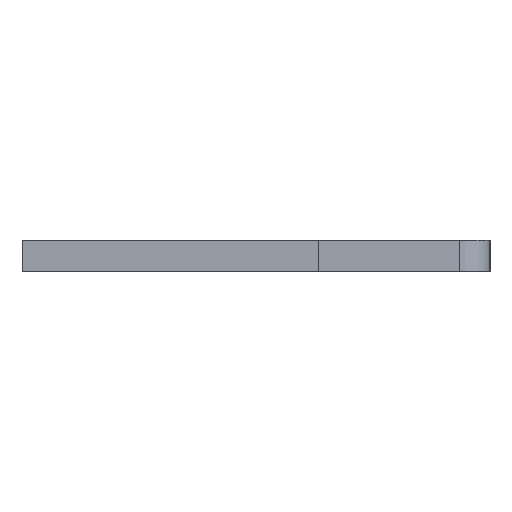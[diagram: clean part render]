
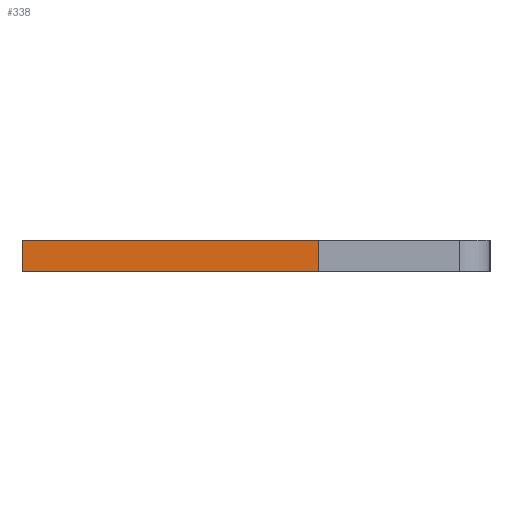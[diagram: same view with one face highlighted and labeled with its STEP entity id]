
A CAD part, left-side view. The second image highlights one B-rep face of the part: STEP entity #338.
In plain terms, the highlighted face is planar.
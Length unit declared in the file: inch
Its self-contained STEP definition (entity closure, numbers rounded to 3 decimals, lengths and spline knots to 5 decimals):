
#32 = LINE ( 'NONE', #143, #63 ) ;
#63 = VECTOR ( 'NONE', #862, 39.37008 ) ;
#90 = PLANE ( 'NONE',  #142 ) ;
#142 = AXIS2_PLACEMENT_3D ( 'NONE', #460, #455, #638 ) ;
#143 = CARTESIAN_POINT ( 'NONE',  ( 0.01, -0.04, -0.04 ) ) ;
#186 = CARTESIAN_POINT ( 'NONE',  ( 0.01, 0.15, -0.04 ) ) ;
#319 = VERTEX_POINT ( 'NONE', #376 ) ;
#338 = ADVANCED_FACE ( 'NONE', ( #926 ), #90, .F. ) ;
#369 = VERTEX_POINT ( 'NONE', #722 ) ;
#376 = CARTESIAN_POINT ( 'NONE',  ( -0.01, -0.04, -0.04 ) ) ;
#380 = CARTESIAN_POINT ( 'NONE',  ( 0.01, 0.15, -0.04 ) ) ;
#418 = CARTESIAN_POINT ( 'NONE',  ( -0.01, 0.15, -0.04 ) ) ;
#434 = LINE ( 'NONE', #1019, #910 ) ;
#449 = VERTEX_POINT ( 'NONE', #186 ) ;
#455 = DIRECTION ( 'NONE',  ( 0., 0., 1. ) ) ;
#460 = CARTESIAN_POINT ( 'NONE',  ( 0.01, 0.15, -0.04 ) ) ;
#467 = EDGE_LOOP ( 'NONE', ( #878, #928, #491, #912 ) ) ;
#474 = EDGE_CURVE ( 'NONE', #449, #535, #655, .T. ) ;
#475 = DIRECTION ( 'NONE',  ( 0., 1., 0. ) ) ;
#491 = ORIENTED_EDGE ( 'NONE', *, *, #712, .F. ) ;
#508 = DIRECTION ( 'NONE',  ( 0., 1., 0. ) ) ;
#535 = VERTEX_POINT ( 'NONE', #933 ) ;
#638 = DIRECTION ( 'NONE',  ( 1., 0., 0. ) ) ;
#655 = LINE ( 'NONE', #380, #1039 ) ;
#712 = EDGE_CURVE ( 'NONE', #369, #449, #434, .T. ) ;
#719 = LINE ( 'NONE', #418, #924 ) ;
#722 = CARTESIAN_POINT ( 'NONE',  ( 0.01, -0.04, -0.04 ) ) ;
#816 = EDGE_CURVE ( 'NONE', #319, #535, #719, .T. ) ;
#830 = DIRECTION ( 'NONE',  ( -1., 0., 0. ) ) ;
#862 = DIRECTION ( 'NONE',  ( -1., 0., 0. ) ) ;
#868 = EDGE_CURVE ( 'NONE', #369, #319, #32, .T. ) ;
#878 = ORIENTED_EDGE ( 'NONE', *, *, #816, .T. ) ;
#910 = VECTOR ( 'NONE', #475, 39.37008 ) ;
#912 = ORIENTED_EDGE ( 'NONE', *, *, #868, .T. ) ;
#924 = VECTOR ( 'NONE', #508, 39.37008 ) ;
#926 = FACE_OUTER_BOUND ( 'NONE', #467, .T. ) ;
#928 = ORIENTED_EDGE ( 'NONE', *, *, #474, .F. ) ;
#933 = CARTESIAN_POINT ( 'NONE',  ( -0.01, 0.15, -0.04 ) ) ;
#1019 = CARTESIAN_POINT ( 'NONE',  ( 0.01, 0.15, -0.04 ) ) ;
#1039 = VECTOR ( 'NONE', #830, 39.37008 ) ;
